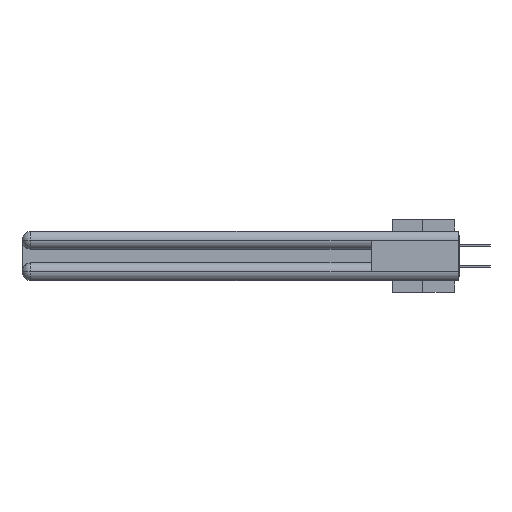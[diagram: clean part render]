
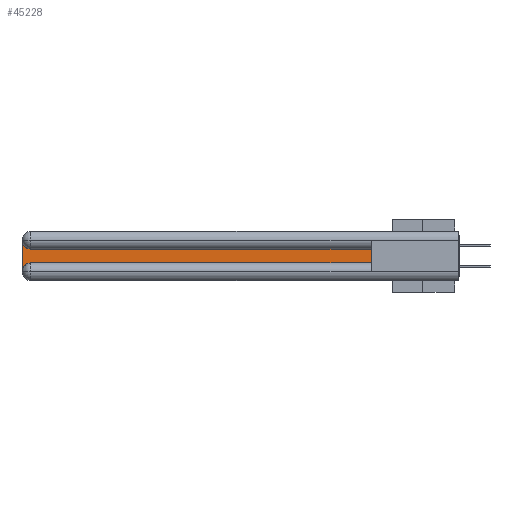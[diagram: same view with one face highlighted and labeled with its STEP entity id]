
A CAD part, left-side view. The second image highlights one B-rep face of the part: STEP entity #45228.
In plain terms, the highlighted planar face has unit normal (-1, 0, 0).
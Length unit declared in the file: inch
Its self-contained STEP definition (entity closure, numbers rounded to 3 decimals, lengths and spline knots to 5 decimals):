
#288 = DIRECTION ( 'NONE',  ( 0., -1., 0. ) ) ;
#3118 = EDGE_LOOP ( 'NONE', ( #11643, #9805, #19586, #26843, #40396, #15923 ) ) ;
#3143 = CARTESIAN_POINT ( 'NONE',  ( 0.075, 2.94, -0.2175 ) ) ;
#3637 = CARTESIAN_POINT ( 'NONE',  ( 0.075, 0.6, -0.2175 ) ) ;
#4212 = VECTOR ( 'NONE', #17499, 39.37008 ) ;
#5429 = LINE ( 'NONE', #41510, #34943 ) ;
#5583 = PLANE ( 'NONE',  #19745 ) ;
#6971 = CARTESIAN_POINT ( 'NONE',  ( 0.075, 0.6, -0.1225 ) ) ;
#9805 = ORIENTED_EDGE ( 'NONE', *, *, #29895, .T. ) ;
#9936 = CARTESIAN_POINT ( 'NONE',  ( 0.075, 2.94, -0.2775 ) ) ;
#10391 = EDGE_CURVE ( 'NONE', #20048, #45878, #43704, .T. ) ;
#11643 = ORIENTED_EDGE ( 'NONE', *, *, #32007, .T. ) ;
#11868 = VECTOR ( 'NONE', #288, 39.37008 ) ;
#13117 = CIRCLE ( 'NONE', #29189, 0.06 ) ;
#13488 = DIRECTION ( 'NONE',  ( 1., 0., 0. ) ) ;
#14273 = CARTESIAN_POINT ( 'NONE',  ( 0.075, 0.6, -0.2175 ) ) ;
#14463 = CARTESIAN_POINT ( 'NONE',  ( 0.075, 0.6, -0.2175 ) ) ;
#15186 = LINE ( 'NONE', #14273, #11868 ) ;
#15923 = ORIENTED_EDGE ( 'NONE', *, *, #10391, .T. ) ;
#16685 = VERTEX_POINT ( 'NONE', #36283 ) ;
#17133 = FACE_OUTER_BOUND ( 'NONE', #3118, .T. ) ;
#17401 = CARTESIAN_POINT ( 'NONE',  ( 0.075, 3., -0.2175 ) ) ;
#17499 = DIRECTION ( 'NONE',  ( 0., 0., 1. ) ) ;
#17961 = CARTESIAN_POINT ( 'NONE',  ( 0.075, 2.94, -0.1225 ) ) ;
#19586 = ORIENTED_EDGE ( 'NONE', *, *, #22872, .T. ) ;
#19745 = AXIS2_PLACEMENT_3D ( 'NONE', #20348, #20193, #37784 ) ;
#20048 = VERTEX_POINT ( 'NONE', #14463 ) ;
#20193 = DIRECTION ( 'NONE',  ( 1., 0., 0. ) ) ;
#20348 = CARTESIAN_POINT ( 'NONE',  ( 0.075, 3., -0.1225 ) ) ;
#22533 = VERTEX_POINT ( 'NONE', #3143 ) ;
#22572 = LINE ( 'NONE', #17401, #42620 ) ;
#22872 = EDGE_CURVE ( 'NONE', #35168, #16685, #22572, .T. ) ;
#23224 = EDGE_CURVE ( 'NONE', #16685, #22533, #13117, .T. ) ;
#24537 = EDGE_CURVE ( 'NONE', #22533, #20048, #15186, .T. ) ;
#24889 = CARTESIAN_POINT ( 'NONE',  ( 0.075, 3., -0.0625 ) ) ;
#26843 = ORIENTED_EDGE ( 'NONE', *, *, #23224, .T. ) ;
#29189 = AXIS2_PLACEMENT_3D ( 'NONE', #9936, #13488, #38368 ) ;
#29895 = EDGE_CURVE ( 'NONE', #36246, #35168, #32164, .T. ) ;
#32007 = EDGE_CURVE ( 'NONE', #45878, #36246, #5429, .T. ) ;
#32164 = CIRCLE ( 'NONE', #38005, 0.06 ) ;
#33599 = DIRECTION ( 'NONE',  ( 1., 0., 0. ) ) ;
#34943 = VECTOR ( 'NONE', #45684, 39.37008 ) ;
#35168 = VERTEX_POINT ( 'NONE', #24889 ) ;
#36246 = VERTEX_POINT ( 'NONE', #17961 ) ;
#36283 = CARTESIAN_POINT ( 'NONE',  ( 0.075, 3., -0.2775 ) ) ;
#37032 = CARTESIAN_POINT ( 'NONE',  ( 0.075, 2.94, -0.0625 ) ) ;
#37784 = DIRECTION ( 'NONE',  ( 0., 0., -1. ) ) ;
#38005 = AXIS2_PLACEMENT_3D ( 'NONE', #37032, #33599, #44000 ) ;
#38368 = DIRECTION ( 'NONE',  ( 0., 0., -1. ) ) ;
#40396 = ORIENTED_EDGE ( 'NONE', *, *, #24537, .T. ) ;
#41510 = CARTESIAN_POINT ( 'NONE',  ( 0.075, 0.6, -0.1225 ) ) ;
#42620 = VECTOR ( 'NONE', #45845, 39.37008 ) ;
#43704 = LINE ( 'NONE', #3637, #4212 ) ;
#44000 = DIRECTION ( 'NONE',  ( 0., 0., -1. ) ) ;
#45228 = ADVANCED_FACE ( 'NONE', ( #17133 ), #5583, .F. ) ;
#45684 = DIRECTION ( 'NONE',  ( 0., 1., 0. ) ) ;
#45845 = DIRECTION ( 'NONE',  ( 0., 0., -1. ) ) ;
#45878 = VERTEX_POINT ( 'NONE', #6971 ) ;
